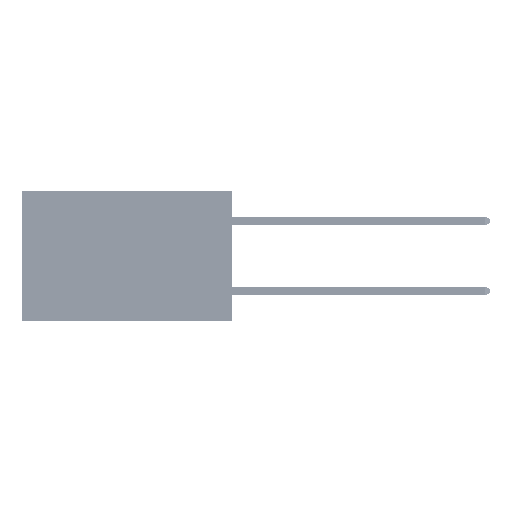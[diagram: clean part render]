
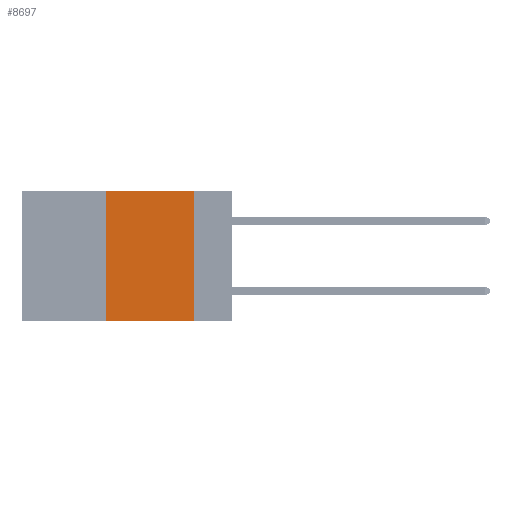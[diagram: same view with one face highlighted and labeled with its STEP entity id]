
A CAD part, left-side view. The second image highlights one B-rep face of the part: STEP entity #8697.
In plain terms, the highlighted planar face has unit normal (-1, 0, 0).
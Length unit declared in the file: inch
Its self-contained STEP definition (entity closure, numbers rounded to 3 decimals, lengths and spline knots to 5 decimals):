
#514 = CARTESIAN_POINT ( 'NONE',  ( 0., 0.11, 0. ) ) ;
#3660 = EDGE_CURVE ( 'NONE', #14707, #8718, #31193, .T. ) ;
#3722 = VECTOR ( 'NONE', #33817, 39.37008 ) ;
#5838 = CARTESIAN_POINT ( 'NONE',  ( 0., 0.6, 0. ) ) ;
#6814 = VECTOR ( 'NONE', #23734, 39.37008 ) ;
#8697 = ADVANCED_FACE ( 'NONE', ( #41738 ), #21844, .F. ) ;
#8718 = VERTEX_POINT ( 'NONE', #44380 ) ;
#9077 = CARTESIAN_POINT ( 'NONE',  ( 0., 0.11, 0. ) ) ;
#10246 = LINE ( 'NONE', #35912, #25300 ) ;
#11484 = VERTEX_POINT ( 'NONE', #26908 ) ;
#13627 = DIRECTION ( 'NONE',  ( 1., 0., 0. ) ) ;
#13884 = EDGE_CURVE ( 'NONE', #41137, #8718, #45325, .T. ) ;
#14707 = VERTEX_POINT ( 'NONE', #29026 ) ;
#15706 = EDGE_CURVE ( 'NONE', #11484, #41137, #10246, .T. ) ;
#21844 = PLANE ( 'NONE',  #47062 ) ;
#22195 = CARTESIAN_POINT ( 'NONE',  ( 0., 0.36, 0. ) ) ;
#22567 = CARTESIAN_POINT ( 'NONE',  ( 0., 0.6, -0.37 ) ) ;
#22989 = LINE ( 'NONE', #22195, #3722 ) ;
#23734 = DIRECTION ( 'NONE',  ( 0., 0., -1. ) ) ;
#23952 = VECTOR ( 'NONE', #34514, 39.37008 ) ;
#25300 = VECTOR ( 'NONE', #39784, 39.37008 ) ;
#26908 = CARTESIAN_POINT ( 'NONE',  ( 0., 0.36, 0. ) ) ;
#27323 = EDGE_LOOP ( 'NONE', ( #35809, #46005, #40710, #45387 ) ) ;
#29026 = CARTESIAN_POINT ( 'NONE',  ( 0., 0.36, -0.37 ) ) ;
#31193 = LINE ( 'NONE', #22567, #23952 ) ;
#33817 = DIRECTION ( 'NONE',  ( 0., 0., 1. ) ) ;
#34514 = DIRECTION ( 'NONE',  ( 0., -1., 0. ) ) ;
#35809 = ORIENTED_EDGE ( 'NONE', *, *, #13884, .F. ) ;
#35912 = CARTESIAN_POINT ( 'NONE',  ( 0., 0.6, 0. ) ) ;
#38183 = EDGE_CURVE ( 'NONE', #14707, #11484, #22989, .T. ) ;
#39784 = DIRECTION ( 'NONE',  ( 0., -1., 0. ) ) ;
#40493 = DIRECTION ( 'NONE',  ( 0., 0., -1. ) ) ;
#40710 = ORIENTED_EDGE ( 'NONE', *, *, #38183, .F. ) ;
#41137 = VERTEX_POINT ( 'NONE', #9077 ) ;
#41738 = FACE_OUTER_BOUND ( 'NONE', #27323, .T. ) ;
#44380 = CARTESIAN_POINT ( 'NONE',  ( 0., 0.11, -0.37 ) ) ;
#45325 = LINE ( 'NONE', #514, #6814 ) ;
#45387 = ORIENTED_EDGE ( 'NONE', *, *, #3660, .T. ) ;
#46005 = ORIENTED_EDGE ( 'NONE', *, *, #15706, .F. ) ;
#47062 = AXIS2_PLACEMENT_3D ( 'NONE', #5838, #13627, #40493 ) ;
